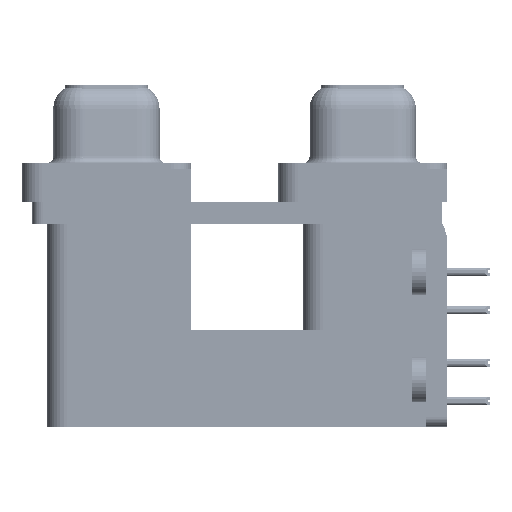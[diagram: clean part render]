
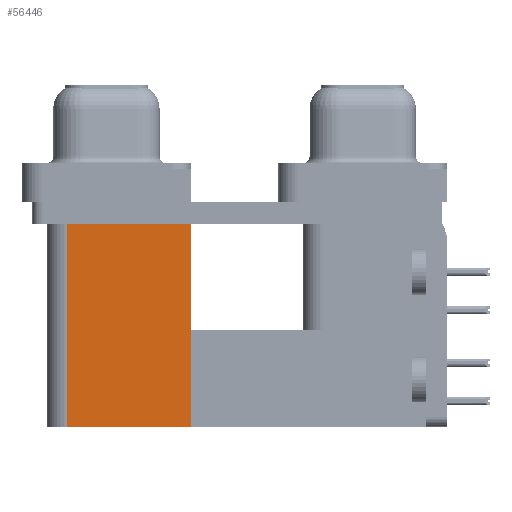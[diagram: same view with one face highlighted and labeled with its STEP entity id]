
A CAD part, left-side view. The second image highlights one B-rep face of the part: STEP entity #56446.
In plain terms, the highlighted planar face has unit normal (-1, 0, 0).
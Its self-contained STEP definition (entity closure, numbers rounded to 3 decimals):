
#1102 = VECTOR ( 'NONE', #11615, 1000. ) ;
#1745 = CARTESIAN_POINT ( 'NONE',  ( 3.7, 12.775, -2.5 ) ) ;
#5842 = LINE ( 'NONE', #21742, #61950 ) ;
#6205 = LINE ( 'NONE', #1745, #1102 ) ;
#6520 = CARTESIAN_POINT ( 'NONE',  ( 3.7, 21.975, -2.5 ) ) ;
#7030 = VERTEX_POINT ( 'NONE', #58157 ) ;
#7279 = PLANE ( 'NONE',  #26548 ) ;
#8129 = VECTOR ( 'NONE', #13789, 1000. ) ;
#8522 = EDGE_CURVE ( 'NONE', #7030, #21767, #38453, .T. ) ;
#9005 = LINE ( 'NONE', #38958, #8129 ) ;
#11615 = DIRECTION ( 'NONE',  ( 0., 1., 0. ) ) ;
#12699 = DIRECTION ( 'NONE',  ( 0., 1., 0. ) ) ;
#13249 = VECTOR ( 'NONE', #42312, 1000. ) ;
#13275 = CARTESIAN_POINT ( 'NONE',  ( 3.7, 12.775, -2.5 ) ) ;
#13789 = DIRECTION ( 'NONE',  ( 0., 0., 1. ) ) ;
#13933 = CARTESIAN_POINT ( 'NONE',  ( 3.7, 12.775, -19.2 ) ) ;
#17794 = DIRECTION ( 'NONE',  ( 1., 0., 0. ) ) ;
#21110 = DIRECTION ( 'NONE',  ( 0., 1., 0. ) ) ;
#21742 = CARTESIAN_POINT ( 'NONE',  ( 3.7, 12.775, -19.2 ) ) ;
#21767 = VERTEX_POINT ( 'NONE', #13275 ) ;
#24953 = EDGE_LOOP ( 'NONE', ( #57234, #50480, #51645, #41863 ) ) ;
#26548 = AXIS2_PLACEMENT_3D ( 'NONE', #55397, #17794, #12699 ) ;
#30360 = CARTESIAN_POINT ( 'NONE',  ( 3.7, 21.975, -19.2 ) ) ;
#38453 = LINE ( 'NONE', #13933, #13249 ) ;
#38958 = CARTESIAN_POINT ( 'NONE',  ( 3.7, 21.975, -19.2 ) ) ;
#41478 = VERTEX_POINT ( 'NONE', #6520 ) ;
#41863 = ORIENTED_EDGE ( 'NONE', *, *, #8522, .T. ) ;
#42312 = DIRECTION ( 'NONE',  ( 0., 0., 1. ) ) ;
#45853 = FACE_OUTER_BOUND ( 'NONE', #24953, .T. ) ;
#50480 = ORIENTED_EDGE ( 'NONE', *, *, #50813, .F. ) ;
#50813 = EDGE_CURVE ( 'NONE', #58700, #41478, #9005, .T. ) ;
#51645 = ORIENTED_EDGE ( 'NONE', *, *, #54074, .F. ) ;
#51824 = EDGE_CURVE ( 'NONE', #21767, #41478, #6205, .T. ) ;
#54074 = EDGE_CURVE ( 'NONE', #7030, #58700, #5842, .T. ) ;
#55397 = CARTESIAN_POINT ( 'NONE',  ( 3.7, 12.775, -19.2 ) ) ;
#56446 = ADVANCED_FACE ( 'NONE', ( #45853 ), #7279, .F. ) ;
#57234 = ORIENTED_EDGE ( 'NONE', *, *, #51824, .T. ) ;
#58157 = CARTESIAN_POINT ( 'NONE',  ( 3.7, 12.775, -19.2 ) ) ;
#58700 = VERTEX_POINT ( 'NONE', #30360 ) ;
#61950 = VECTOR ( 'NONE', #21110, 1000. ) ;
